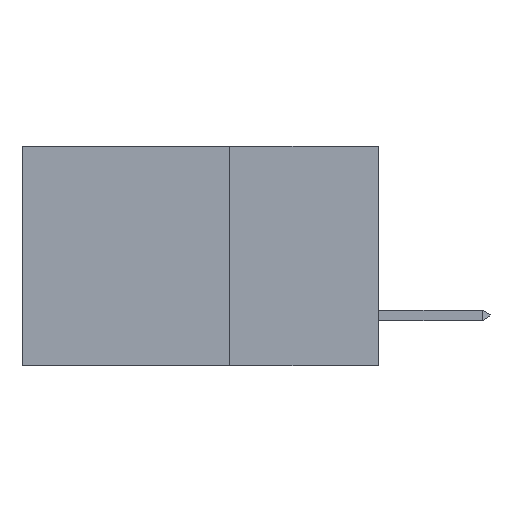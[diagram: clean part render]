
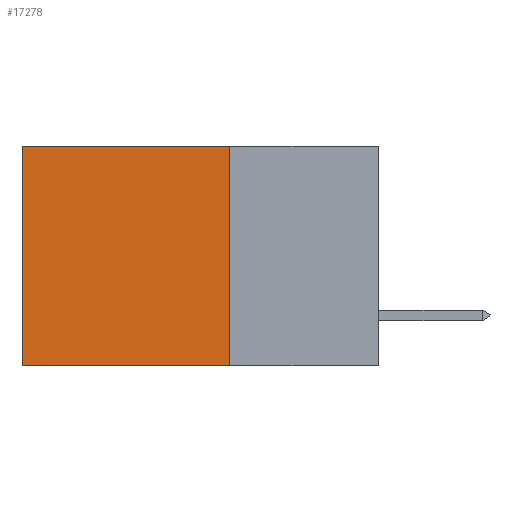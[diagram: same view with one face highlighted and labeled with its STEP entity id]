
A CAD part, left-side view. The second image highlights one B-rep face of the part: STEP entity #17278.
In plain terms, the highlighted planar face has unit normal (-1, 0, 0).
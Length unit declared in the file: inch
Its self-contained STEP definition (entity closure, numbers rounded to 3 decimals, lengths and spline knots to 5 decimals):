
#1511 = EDGE_CURVE ( 'NONE', #4804, #11385, #18467, .T. ) ;
#1781 = FACE_OUTER_BOUND ( 'NONE', #11496, .T. ) ;
#1846 = AXIS2_PLACEMENT_3D ( 'NONE', #14016, #1902, #21420 ) ;
#1902 = DIRECTION ( 'NONE',  ( 1., 0., 0. ) ) ;
#2512 = CARTESIAN_POINT ( 'NONE',  ( 0.2615, 0.6, -0.37 ) ) ;
#4804 = VERTEX_POINT ( 'NONE', #16382 ) ;
#4885 = ORIENTED_EDGE ( 'NONE', *, *, #1511, .T. ) ;
#5241 = CARTESIAN_POINT ( 'NONE',  ( 0.2615, 0.25, 0. ) ) ;
#5359 = LINE ( 'NONE', #5241, #6997 ) ;
#6135 = DIRECTION ( 'NONE',  ( 0., 0., -1. ) ) ;
#6183 = VERTEX_POINT ( 'NONE', #9251 ) ;
#6473 = CARTESIAN_POINT ( 'NONE',  ( 0.2615, 0.25, -0.37 ) ) ;
#6997 = VECTOR ( 'NONE', #19558, 39.37008 ) ;
#7264 = PLANE ( 'NONE',  #1846 ) ;
#7451 = VECTOR ( 'NONE', #18059, 39.37008 ) ;
#9251 = CARTESIAN_POINT ( 'NONE',  ( 0.2615, 0.25, 0. ) ) ;
#10983 = CARTESIAN_POINT ( 'NONE',  ( 0.2615, 0.25, -0.37 ) ) ;
#11349 = EDGE_CURVE ( 'NONE', #6183, #13822, #13690, .T. ) ;
#11385 = VERTEX_POINT ( 'NONE', #17404 ) ;
#11496 = EDGE_LOOP ( 'NONE', ( #4885, #12247, #18861, #14863 ) ) ;
#11938 = DIRECTION ( 'NONE',  ( 0., 0., -1. ) ) ;
#12247 = ORIENTED_EDGE ( 'NONE', *, *, #16128, .F. ) ;
#12362 = VECTOR ( 'NONE', #6135, 39.37008 ) ;
#13192 = EDGE_CURVE ( 'NONE', #6183, #4804, #5359, .T. ) ;
#13690 = LINE ( 'NONE', #6473, #15139 ) ;
#13822 = VERTEX_POINT ( 'NONE', #20796 ) ;
#14016 = CARTESIAN_POINT ( 'NONE',  ( 0.2615, 0.25, -0.37 ) ) ;
#14863 = ORIENTED_EDGE ( 'NONE', *, *, #13192, .T. ) ;
#15139 = VECTOR ( 'NONE', #11938, 39.37008 ) ;
#16128 = EDGE_CURVE ( 'NONE', #13822, #11385, #18175, .T. ) ;
#16382 = CARTESIAN_POINT ( 'NONE',  ( 0.2615, 0.6, 0. ) ) ;
#17278 = ADVANCED_FACE ( 'NONE', ( #1781 ), #7264, .F. ) ;
#17404 = CARTESIAN_POINT ( 'NONE',  ( 0.2615, 0.6, -0.37 ) ) ;
#18059 = DIRECTION ( 'NONE',  ( 0., 1., 0. ) ) ;
#18175 = LINE ( 'NONE', #10983, #7451 ) ;
#18467 = LINE ( 'NONE', #2512, #12362 ) ;
#18861 = ORIENTED_EDGE ( 'NONE', *, *, #11349, .F. ) ;
#19558 = DIRECTION ( 'NONE',  ( 0., 1., 0. ) ) ;
#20796 = CARTESIAN_POINT ( 'NONE',  ( 0.2615, 0.25, -0.37 ) ) ;
#21420 = DIRECTION ( 'NONE',  ( 0., 0., -1. ) ) ;
